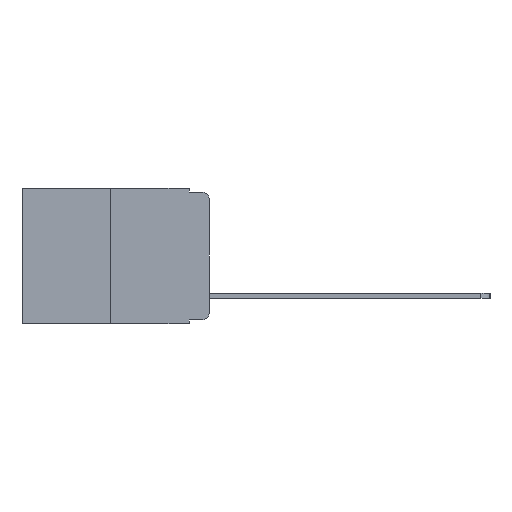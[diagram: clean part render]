
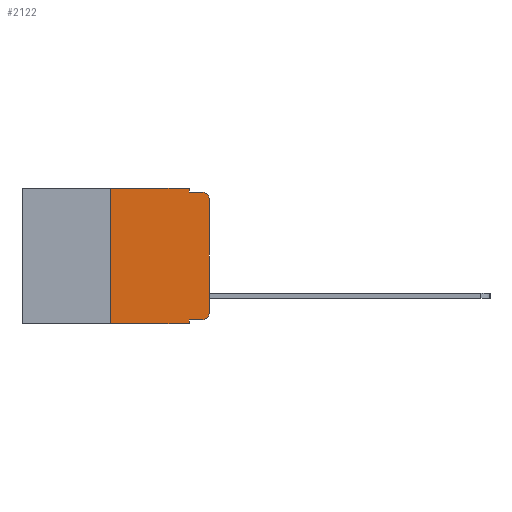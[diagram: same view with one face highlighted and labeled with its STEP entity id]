
A CAD part, left-side view. The second image highlights one B-rep face of the part: STEP entity #2122.
In plain terms, the highlighted planar face has unit normal (-1, 0, 0).
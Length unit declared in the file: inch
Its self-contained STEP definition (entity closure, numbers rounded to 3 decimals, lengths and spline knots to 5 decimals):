
#985 = CARTESIAN_POINT ( 'NONE',  ( 0., 0.051, -0.333 ) ) ;
#1013 = PLANE ( 'NONE',  #15872 ) ;
#1287 = LINE ( 'NONE', #1623, #16360 ) ;
#1333 = CARTESIAN_POINT ( 'NONE',  ( 0., 0., -0.313 ) ) ;
#1474 = ORIENTED_EDGE ( 'NONE', *, *, #12734, .F. ) ;
#1623 = CARTESIAN_POINT ( 'NONE',  ( 0., 0., 0. ) ) ;
#1740 = ORIENTED_EDGE ( 'NONE', *, *, #15143, .T. ) ;
#1770 = EDGE_LOOP ( 'NONE', ( #1740, #8087, #7199, #1474, #8210, #9414, #6564, #6693, #4254, #2356 ) ) ;
#1819 = VERTEX_POINT ( 'NONE', #12049 ) ;
#1877 = DIRECTION ( 'NONE',  ( 0., 0., -1. ) ) ;
#1931 = LINE ( 'NONE', #15722, #13131 ) ;
#1936 = EDGE_CURVE ( 'NONE', #8281, #2334, #6878, .T. ) ;
#2122 = ADVANCED_FACE ( 'NONE', ( #4476 ), #1013, .F. ) ;
#2334 = VERTEX_POINT ( 'NONE', #8599 ) ;
#2356 = ORIENTED_EDGE ( 'NONE', *, *, #15025, .T. ) ;
#2443 = EDGE_CURVE ( 'NONE', #17461, #1819, #6862, .T. ) ;
#2967 = CARTESIAN_POINT ( 'NONE',  ( 0., 0.473, -0.343 ) ) ;
#3145 = DIRECTION ( 'NONE',  ( 0., 0., 1. ) ) ;
#3215 = LINE ( 'NONE', #2967, #6838 ) ;
#4149 = VERTEX_POINT ( 'NONE', #1333 ) ;
#4254 = ORIENTED_EDGE ( 'NONE', *, *, #16892, .T. ) ;
#4476 = FACE_OUTER_BOUND ( 'NONE', #1770, .T. ) ;
#4665 = CIRCLE ( 'NONE', #17435, 0.02 ) ;
#4895 = CARTESIAN_POINT ( 'NONE',  ( 0., 0.051, -0.01 ) ) ;
#4948 = CARTESIAN_POINT ( 'NONE',  ( 0., 0.051, -0.343 ) ) ;
#5603 = LINE ( 'NONE', #15636, #16566 ) ;
#6070 = EDGE_CURVE ( 'NONE', #8281, #13646, #3215, .T. ) ;
#6564 = ORIENTED_EDGE ( 'NONE', *, *, #6070, .T. ) ;
#6569 = CARTESIAN_POINT ( 'NONE',  ( 0., 0., -0.03 ) ) ;
#6693 = ORIENTED_EDGE ( 'NONE', *, *, #18724, .F. ) ;
#6722 = CARTESIAN_POINT ( 'NONE',  ( 0., 0.02, -0.03 ) ) ;
#6838 = VECTOR ( 'NONE', #11576, 39.37008 ) ;
#6862 = LINE ( 'NONE', #4895, #10213 ) ;
#6878 = LINE ( 'NONE', #10104, #14893 ) ;
#7013 = CARTESIAN_POINT ( 'NONE',  ( 0., 0.051, -0.01 ) ) ;
#7199 = ORIENTED_EDGE ( 'NONE', *, *, #2443, .F. ) ;
#7403 = DIRECTION ( 'NONE',  ( 0., -1., 0. ) ) ;
#8087 = ORIENTED_EDGE ( 'NONE', *, *, #9462, .T. ) ;
#8201 = DIRECTION ( 'NONE',  ( 0., 0., -1. ) ) ;
#8210 = ORIENTED_EDGE ( 'NONE', *, *, #18797, .F. ) ;
#8281 = VERTEX_POINT ( 'NONE', #15249 ) ;
#8599 = CARTESIAN_POINT ( 'NONE',  ( 0., 0.25, 0. ) ) ;
#8885 = CARTESIAN_POINT ( 'NONE',  ( 0., 0.02, -0.313 ) ) ;
#9414 = ORIENTED_EDGE ( 'NONE', *, *, #1936, .F. ) ;
#9462 = EDGE_CURVE ( 'NONE', #9986, #1819, #12262, .T. ) ;
#9648 = VERTEX_POINT ( 'NONE', #985 ) ;
#9986 = VERTEX_POINT ( 'NONE', #6569 ) ;
#10044 = VECTOR ( 'NONE', #10216, 39.37008 ) ;
#10104 = CARTESIAN_POINT ( 'NONE',  ( 0., 0.25, 0. ) ) ;
#10213 = VECTOR ( 'NONE', #10495, 39.37008 ) ;
#10216 = DIRECTION ( 'NONE',  ( 0., 0., -1. ) ) ;
#10266 = DIRECTION ( 'NONE',  ( 0., 0., 1. ) ) ;
#10297 = DIRECTION ( 'NONE',  ( 0., 0., -1. ) ) ;
#10398 = VERTEX_POINT ( 'NONE', #11772 ) ;
#10495 = DIRECTION ( 'NONE',  ( 0., -1., 0. ) ) ;
#10661 = CARTESIAN_POINT ( 'NONE',  ( 0., 0.02, -0.333 ) ) ;
#11576 = DIRECTION ( 'NONE',  ( 0., -1., 0. ) ) ;
#11772 = CARTESIAN_POINT ( 'NONE',  ( 0., 0.051, 0. ) ) ;
#12049 = CARTESIAN_POINT ( 'NONE',  ( 0., 0.02, -0.01 ) ) ;
#12262 = CIRCLE ( 'NONE', #13805, 0.02 ) ;
#12734 = EDGE_CURVE ( 'NONE', #10398, #17461, #13795, .T. ) ;
#13131 = VECTOR ( 'NONE', #17152, 39.37008 ) ;
#13646 = VERTEX_POINT ( 'NONE', #4948 ) ;
#13795 = LINE ( 'NONE', #14416, #10044 ) ;
#13805 = AXIS2_PLACEMENT_3D ( 'NONE', #6722, #16639, #8201 ) ;
#14416 = CARTESIAN_POINT ( 'NONE',  ( 0., 0.051, 0. ) ) ;
#14893 = VECTOR ( 'NONE', #10266, 39.37008 ) ;
#15025 = EDGE_CURVE ( 'NONE', #17762, #4149, #4665, .T. ) ;
#15143 = EDGE_CURVE ( 'NONE', #4149, #9986, #1287, .T. ) ;
#15249 = CARTESIAN_POINT ( 'NONE',  ( 0., 0.25, -0.343 ) ) ;
#15587 = VECTOR ( 'NONE', #7403, 39.37008 ) ;
#15636 = CARTESIAN_POINT ( 'NONE',  ( 0., 0.051, -0.333 ) ) ;
#15722 = CARTESIAN_POINT ( 'NONE',  ( 0., 0.051, 0. ) ) ;
#15872 = AXIS2_PLACEMENT_3D ( 'NONE', #16350, #16520, #1877 ) ;
#16025 = LINE ( 'NONE', #18630, #15587 ) ;
#16350 = CARTESIAN_POINT ( 'NONE',  ( 0., 0.473, 0. ) ) ;
#16360 = VECTOR ( 'NONE', #3145, 39.37008 ) ;
#16520 = DIRECTION ( 'NONE',  ( 1., 0., 0. ) ) ;
#16566 = VECTOR ( 'NONE', #17061, 39.37008 ) ;
#16639 = DIRECTION ( 'NONE',  ( -1., 0., 0. ) ) ;
#16892 = EDGE_CURVE ( 'NONE', #9648, #17762, #5603, .T. ) ;
#17061 = DIRECTION ( 'NONE',  ( 0., -1., 0. ) ) ;
#17152 = DIRECTION ( 'NONE',  ( 0., 0., -1. ) ) ;
#17435 = AXIS2_PLACEMENT_3D ( 'NONE', #8885, #18691, #10297 ) ;
#17461 = VERTEX_POINT ( 'NONE', #7013 ) ;
#17762 = VERTEX_POINT ( 'NONE', #10661 ) ;
#18630 = CARTESIAN_POINT ( 'NONE',  ( 0., 0.473, 0. ) ) ;
#18691 = DIRECTION ( 'NONE',  ( -1., 0., 0. ) ) ;
#18724 = EDGE_CURVE ( 'NONE', #9648, #13646, #1931, .T. ) ;
#18797 = EDGE_CURVE ( 'NONE', #2334, #10398, #16025, .T. ) ;
